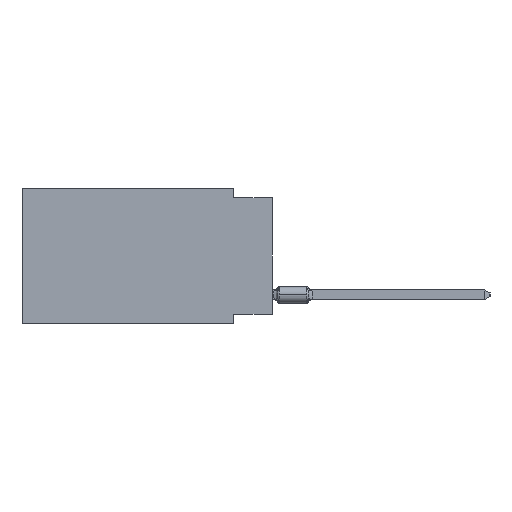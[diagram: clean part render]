
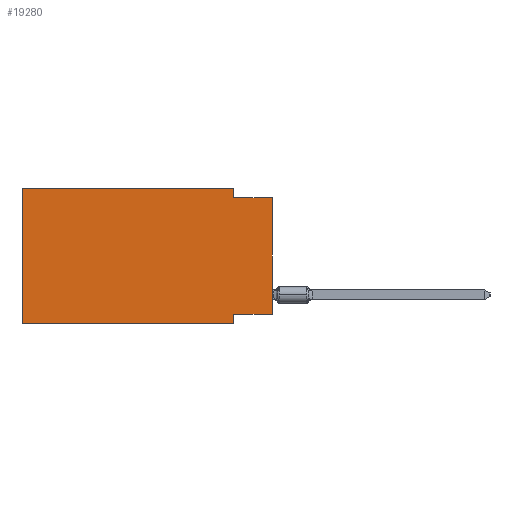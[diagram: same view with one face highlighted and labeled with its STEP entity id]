
A CAD part, left-side view. The second image highlights one B-rep face of the part: STEP entity #19280.
In plain terms, the highlighted planar face has unit normal (-1, 0, 0).
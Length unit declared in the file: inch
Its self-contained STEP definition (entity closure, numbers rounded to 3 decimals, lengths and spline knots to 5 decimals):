
#21 = PLANE ( 'NONE',  #7467 ) ;
#149 = ORIENTED_EDGE ( 'NONE', *, *, #33359, .F. ) ;
#449 = CARTESIAN_POINT ( 'NONE',  ( 0., 0.1, 0. ) ) ;
#482 = VERTEX_POINT ( 'NONE', #21330 ) ;
#1175 = EDGE_CURVE ( 'NONE', #17636, #8543, #3181, .T. ) ;
#1406 = EDGE_CURVE ( 'NONE', #27460, #5562, #22382, .T. ) ;
#1847 = CARTESIAN_POINT ( 'NONE',  ( 0., 0.645, -0.35 ) ) ;
#3181 = LINE ( 'NONE', #18477, #16789 ) ;
#3314 = EDGE_CURVE ( 'NONE', #29550, #17636, #24424, .T. ) ;
#4662 = DIRECTION ( 'NONE',  ( 0., 0., 1. ) ) ;
#4992 = CARTESIAN_POINT ( 'NONE',  ( 0., 0.1, -0.35 ) ) ;
#5562 = VERTEX_POINT ( 'NONE', #4992 ) ;
#6647 = DIRECTION ( 'NONE',  ( 0., -1., 0. ) ) ;
#7272 = EDGE_CURVE ( 'NONE', #17996, #27460, #26839, .T. ) ;
#7467 = AXIS2_PLACEMENT_3D ( 'NONE', #23655, #25843, #10724 ) ;
#8543 = VERTEX_POINT ( 'NONE', #31866 ) ;
#8969 = CARTESIAN_POINT ( 'NONE',  ( 0., 0.645, 0. ) ) ;
#9878 = ORIENTED_EDGE ( 'NONE', *, *, #32407, .T. ) ;
#10149 = VERTEX_POINT ( 'NONE', #30311 ) ;
#10646 = ORIENTED_EDGE ( 'NONE', *, *, #3314, .F. ) ;
#10724 = DIRECTION ( 'NONE',  ( 0., 0., -1. ) ) ;
#11360 = VECTOR ( 'NONE', #32721, 39.37008 ) ;
#11373 = DIRECTION ( 'NONE',  ( 0., 1., 0. ) ) ;
#11792 = LINE ( 'NONE', #22156, #22785 ) ;
#12965 = DIRECTION ( 'NONE',  ( 0., 0., 1. ) ) ;
#14272 = ORIENTED_EDGE ( 'NONE', *, *, #1175, .F. ) ;
#16128 = CARTESIAN_POINT ( 'NONE',  ( 0., 0., -0.325 ) ) ;
#16789 = VECTOR ( 'NONE', #31207, 39.37008 ) ;
#16857 = VECTOR ( 'NONE', #4662, 39.37008 ) ;
#17636 = VERTEX_POINT ( 'NONE', #27969 ) ;
#17996 = VERTEX_POINT ( 'NONE', #18780 ) ;
#18477 = CARTESIAN_POINT ( 'NONE',  ( 0., 0.645, 0. ) ) ;
#18780 = CARTESIAN_POINT ( 'NONE',  ( 0., 0., -0.325 ) ) ;
#19280 = ADVANCED_FACE ( 'NONE', ( #23304 ), #21, .F. ) ;
#19399 = CARTESIAN_POINT ( 'NONE',  ( 0., 0.1, -0.325 ) ) ;
#20267 = EDGE_CURVE ( 'NONE', #8543, #10149, #23735, .T. ) ;
#20952 = EDGE_LOOP ( 'NONE', ( #26110, #149, #28721, #14272, #10646, #9878, #32700, #27497 ) ) ;
#21330 = CARTESIAN_POINT ( 'NONE',  ( 0., 0., -0.025 ) ) ;
#22156 = CARTESIAN_POINT ( 'NONE',  ( 0., 0.645, -0.35 ) ) ;
#22275 = CARTESIAN_POINT ( 'NONE',  ( 0., 0., -0.025 ) ) ;
#22382 = LINE ( 'NONE', #32541, #11360 ) ;
#22458 = LINE ( 'NONE', #22275, #26105 ) ;
#22785 = VECTOR ( 'NONE', #32165, 39.37008 ) ;
#23304 = FACE_OUTER_BOUND ( 'NONE', #20952, .T. ) ;
#23340 = CARTESIAN_POINT ( 'NONE',  ( 0., 0., 0. ) ) ;
#23467 = EDGE_CURVE ( 'NONE', #17996, #482, #28260, .T. ) ;
#23655 = CARTESIAN_POINT ( 'NONE',  ( 0., 0.645, 0. ) ) ;
#23735 = LINE ( 'NONE', #449, #26503 ) ;
#24424 = LINE ( 'NONE', #8969, #16857 ) ;
#25044 = VECTOR ( 'NONE', #12965, 39.37008 ) ;
#25626 = VECTOR ( 'NONE', #11373, 39.37008 ) ;
#25843 = DIRECTION ( 'NONE',  ( 1., 0., 0. ) ) ;
#26105 = VECTOR ( 'NONE', #6647, 39.37008 ) ;
#26110 = ORIENTED_EDGE ( 'NONE', *, *, #23467, .T. ) ;
#26503 = VECTOR ( 'NONE', #31519, 39.37008 ) ;
#26839 = LINE ( 'NONE', #16128, #25626 ) ;
#27460 = VERTEX_POINT ( 'NONE', #19399 ) ;
#27497 = ORIENTED_EDGE ( 'NONE', *, *, #7272, .F. ) ;
#27969 = CARTESIAN_POINT ( 'NONE',  ( 0., 0.645, 0. ) ) ;
#28260 = LINE ( 'NONE', #23340, #25044 ) ;
#28721 = ORIENTED_EDGE ( 'NONE', *, *, #20267, .F. ) ;
#29550 = VERTEX_POINT ( 'NONE', #1847 ) ;
#30311 = CARTESIAN_POINT ( 'NONE',  ( 0., 0.1, -0.025 ) ) ;
#31207 = DIRECTION ( 'NONE',  ( 0., -1., 0. ) ) ;
#31519 = DIRECTION ( 'NONE',  ( 0., 0., -1. ) ) ;
#31866 = CARTESIAN_POINT ( 'NONE',  ( 0., 0.1, 0. ) ) ;
#32165 = DIRECTION ( 'NONE',  ( 0., -1., 0. ) ) ;
#32407 = EDGE_CURVE ( 'NONE', #29550, #5562, #11792, .T. ) ;
#32541 = CARTESIAN_POINT ( 'NONE',  ( 0., 0.1, -0.35 ) ) ;
#32700 = ORIENTED_EDGE ( 'NONE', *, *, #1406, .F. ) ;
#32721 = DIRECTION ( 'NONE',  ( 0., 0., -1. ) ) ;
#33359 = EDGE_CURVE ( 'NONE', #10149, #482, #22458, .T. ) ;
